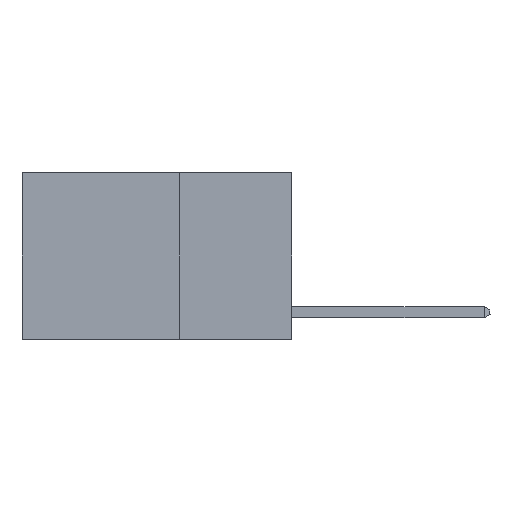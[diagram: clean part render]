
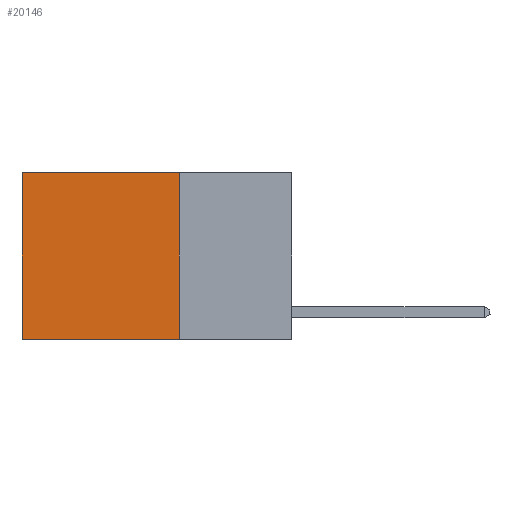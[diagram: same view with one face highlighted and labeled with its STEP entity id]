
A CAD part, left-side view. The second image highlights one B-rep face of the part: STEP entity #20146.
In plain terms, the highlighted planar face has unit normal (-1, 0, 0).
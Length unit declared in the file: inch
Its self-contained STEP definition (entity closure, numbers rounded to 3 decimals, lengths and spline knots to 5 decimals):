
#324 = VECTOR ( 'NONE', #6431, 39.37008 ) ;
#452 = EDGE_CURVE ( 'NONE', #9544, #5906, #4812, .T. ) ;
#486 = VERTEX_POINT ( 'NONE', #4705 ) ;
#667 = CARTESIAN_POINT ( 'NONE',  ( 0.2625, 0.25, -0.37 ) ) ;
#1240 = CARTESIAN_POINT ( 'NONE',  ( 0.2625, 0.25, 0. ) ) ;
#1406 = EDGE_LOOP ( 'NONE', ( #15718, #3239, #5612, #2923 ) ) ;
#1906 = LINE ( 'NONE', #667, #20440 ) ;
#2923 = ORIENTED_EDGE ( 'NONE', *, *, #18101, .T. ) ;
#3194 = DIRECTION ( 'NONE',  ( 0., 0., -1. ) ) ;
#3239 = ORIENTED_EDGE ( 'NONE', *, *, #7686, .F. ) ;
#4705 = CARTESIAN_POINT ( 'NONE',  ( 0.2625, 0.6, -0.37 ) ) ;
#4812 = LINE ( 'NONE', #1240, #12630 ) ;
#4918 = DIRECTION ( 'NONE',  ( 0., 0., -1. ) ) ;
#5053 = AXIS2_PLACEMENT_3D ( 'NONE', #17347, #8815, #18911 ) ;
#5612 = ORIENTED_EDGE ( 'NONE', *, *, #452, .F. ) ;
#5906 = VERTEX_POINT ( 'NONE', #17308 ) ;
#6431 = DIRECTION ( 'NONE',  ( 0., 1., 0. ) ) ;
#7686 = EDGE_CURVE ( 'NONE', #5906, #486, #1906, .T. ) ;
#8815 = DIRECTION ( 'NONE',  ( 1., 0., 0. ) ) ;
#9544 = VERTEX_POINT ( 'NONE', #12399 ) ;
#10164 = PLANE ( 'NONE',  #5053 ) ;
#11588 = CARTESIAN_POINT ( 'NONE',  ( 0.2625, 0.25, 0. ) ) ;
#12399 = CARTESIAN_POINT ( 'NONE',  ( 0.2625, 0.25, 0. ) ) ;
#12630 = VECTOR ( 'NONE', #4918, 39.37008 ) ;
#13251 = VECTOR ( 'NONE', #3194, 39.37008 ) ;
#13477 = CARTESIAN_POINT ( 'NONE',  ( 0.2625, 0.6, 0. ) ) ;
#13847 = FACE_OUTER_BOUND ( 'NONE', #1406, .T. ) ;
#15290 = LINE ( 'NONE', #13477, #13251 ) ;
#15718 = ORIENTED_EDGE ( 'NONE', *, *, #19344, .T. ) ;
#16157 = CARTESIAN_POINT ( 'NONE',  ( 0.2625, 0.6, 0. ) ) ;
#16893 = VERTEX_POINT ( 'NONE', #16157 ) ;
#17308 = CARTESIAN_POINT ( 'NONE',  ( 0.2625, 0.25, -0.37 ) ) ;
#17347 = CARTESIAN_POINT ( 'NONE',  ( 0.2625, 0.25, 0. ) ) ;
#17598 = DIRECTION ( 'NONE',  ( 0., 1., 0. ) ) ;
#18101 = EDGE_CURVE ( 'NONE', #9544, #16893, #20305, .T. ) ;
#18911 = DIRECTION ( 'NONE',  ( 0., 0., -1. ) ) ;
#19344 = EDGE_CURVE ( 'NONE', #16893, #486, #15290, .T. ) ;
#20146 = ADVANCED_FACE ( 'NONE', ( #13847 ), #10164, .F. ) ;
#20305 = LINE ( 'NONE', #11588, #324 ) ;
#20440 = VECTOR ( 'NONE', #17598, 39.37008 ) ;
